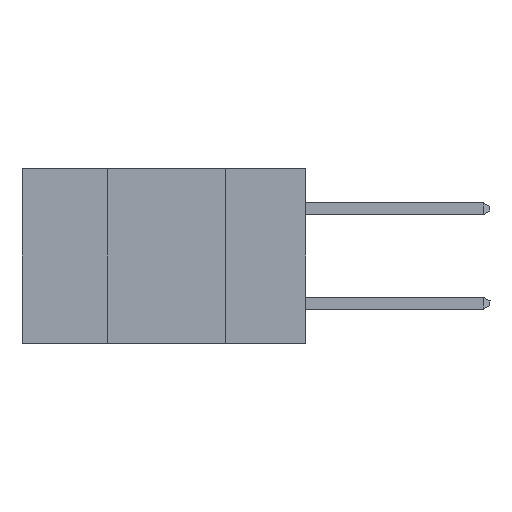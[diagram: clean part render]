
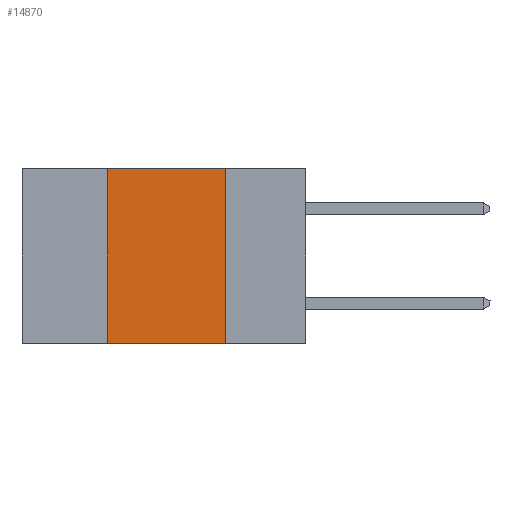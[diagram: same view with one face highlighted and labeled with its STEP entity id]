
A CAD part, left-side view. The second image highlights one B-rep face of the part: STEP entity #14870.
In plain terms, the highlighted planar face has unit normal (-1, 0, 0).
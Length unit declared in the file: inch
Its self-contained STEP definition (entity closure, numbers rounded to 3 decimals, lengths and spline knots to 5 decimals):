
#1538 = CARTESIAN_POINT ( 'NONE',  ( 0., 0.6, -0.37 ) ) ;
#2507 = DIRECTION ( 'NONE',  ( 0., 0., 1. ) ) ;
#3099 = PLANE ( 'NONE',  #19813 ) ;
#4078 = VERTEX_POINT ( 'NONE', #5019 ) ;
#4938 = EDGE_CURVE ( 'NONE', #19605, #4078, #11358, .T. ) ;
#5019 = CARTESIAN_POINT ( 'NONE',  ( 0., 0.17, 0. ) ) ;
#5045 = VERTEX_POINT ( 'NONE', #23650 ) ;
#5077 = VECTOR ( 'NONE', #9942, 39.37008 ) ;
#5515 = CARTESIAN_POINT ( 'NONE',  ( 0., 0.42, -0.37 ) ) ;
#6197 = EDGE_CURVE ( 'NONE', #21254, #19605, #7846, .T. ) ;
#7846 = LINE ( 'NONE', #19147, #20646 ) ;
#7973 = ORIENTED_EDGE ( 'NONE', *, *, #23727, .F. ) ;
#8169 = ORIENTED_EDGE ( 'NONE', *, *, #6197, .F. ) ;
#8692 = ORIENTED_EDGE ( 'NONE', *, *, #11162, .T. ) ;
#8851 = DIRECTION ( 'NONE',  ( 1., 0., 0. ) ) ;
#9942 = DIRECTION ( 'NONE',  ( 0., 0., -1. ) ) ;
#10639 = FACE_OUTER_BOUND ( 'NONE', #18121, .T. ) ;
#11133 = DIRECTION ( 'NONE',  ( 0., -1., 0. ) ) ;
#11162 = EDGE_CURVE ( 'NONE', #21254, #5045, #13319, .T. ) ;
#11358 = LINE ( 'NONE', #23409, #16202 ) ;
#12598 = DIRECTION ( 'NONE',  ( 0., -1., 0. ) ) ;
#13319 = LINE ( 'NONE', #1538, #22360 ) ;
#14870 = ADVANCED_FACE ( 'NONE', ( #10639 ), #3099, .F. ) ;
#15085 = ORIENTED_EDGE ( 'NONE', *, *, #4938, .F. ) ;
#16202 = VECTOR ( 'NONE', #12598, 39.37008 ) ;
#18121 = EDGE_LOOP ( 'NONE', ( #7973, #15085, #8169, #8692 ) ) ;
#19147 = CARTESIAN_POINT ( 'NONE',  ( 0., 0.42, -0.37 ) ) ;
#19605 = VERTEX_POINT ( 'NONE', #21204 ) ;
#19705 = CARTESIAN_POINT ( 'NONE',  ( 0., 0.6, 0. ) ) ;
#19813 = AXIS2_PLACEMENT_3D ( 'NONE', #19705, #8851, #21516 ) ;
#20646 = VECTOR ( 'NONE', #2507, 39.37008 ) ;
#21204 = CARTESIAN_POINT ( 'NONE',  ( 0., 0.42, 0. ) ) ;
#21254 = VERTEX_POINT ( 'NONE', #5515 ) ;
#21516 = DIRECTION ( 'NONE',  ( 0., 0., -1. ) ) ;
#22360 = VECTOR ( 'NONE', #11133, 39.37008 ) ;
#22590 = CARTESIAN_POINT ( 'NONE',  ( 0., 0.17, -0.37 ) ) ;
#23409 = CARTESIAN_POINT ( 'NONE',  ( 0., 0.6, 0. ) ) ;
#23650 = CARTESIAN_POINT ( 'NONE',  ( 0., 0.17, -0.37 ) ) ;
#23727 = EDGE_CURVE ( 'NONE', #4078, #5045, #23895, .T. ) ;
#23895 = LINE ( 'NONE', #22590, #5077 ) ;
